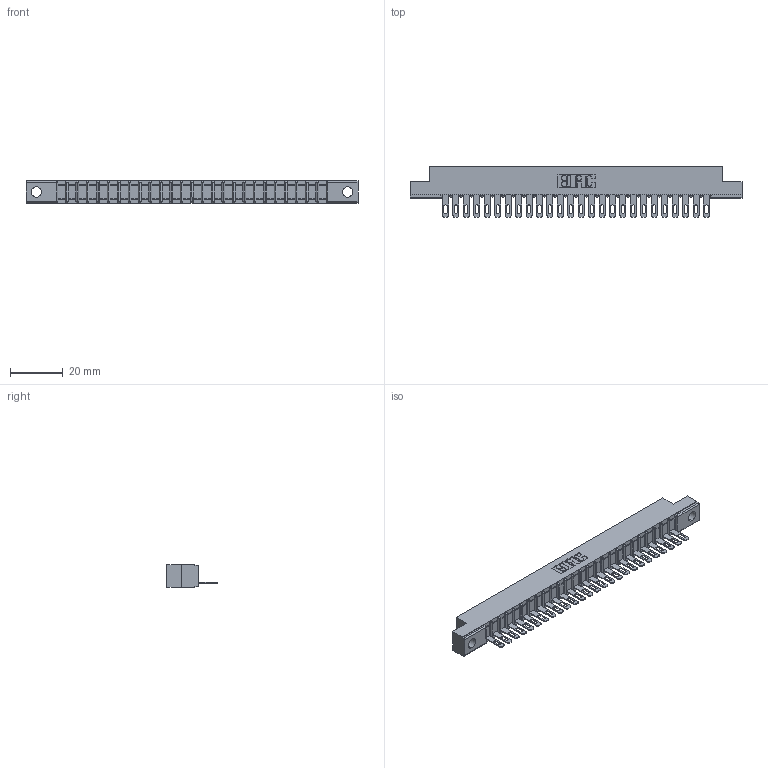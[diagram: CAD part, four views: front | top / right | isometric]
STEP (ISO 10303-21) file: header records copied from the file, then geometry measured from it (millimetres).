
FILE_DESCRIPTION (( 'STEP AP203' ), '1' );
FILE_NAME ('357-026-405-104.STEP', '2020-10-01T16:08:41', ( '' ), ( '' ), 'SwSTEP 2.0', 'SolidWorks 2020', '' );
FILE_SCHEMA (( 'CONFIG_CONTROL_DESIGN' ));
Length unit declared in the file: inch
Products named in the file (3): 307-290-001_505; 307 Part_.156 Dia Mounting Holes; 357-026-405-104
Assembly tree (27 placements, depth 2):
  357-026-405-104
    307 Part_.156 Dia Mounting Holes
    307-290-001_505  x26
Bounding box: 126.03 x 19.18 x 8.71 mm (x, y, z)
Volume: 7876.7 mm3; surface area: 12442.2 mm2
Topology: 27 solids, 27 shells, 1615 faces, 4571 edges, 2938 vertices
Faces by surface type: plane 1020, cylinder 541, sphere 54
Entity records: 24654 total; most frequent: CARTESIAN_POINT 4150, ORIENTED_EDGE 4134, DIRECTION 4039, EDGE_CURVE 2067, VECTOR 1585, LINE 1585, VERTEX_POINT 1338, AXIS2_PLACEMENT_3D 1227
